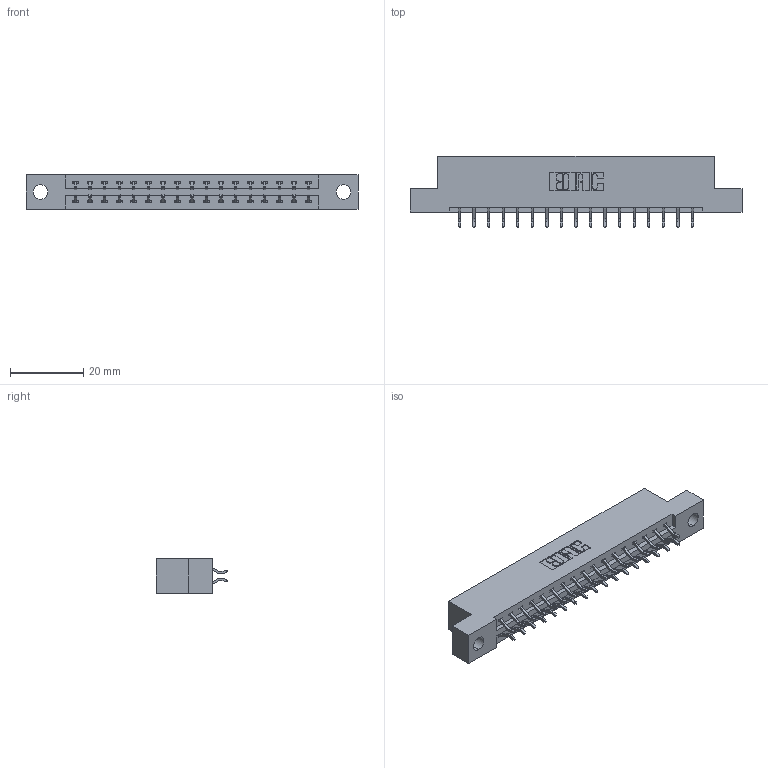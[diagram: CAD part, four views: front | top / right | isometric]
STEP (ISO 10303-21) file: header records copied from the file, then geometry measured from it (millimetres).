
FILE_DESCRIPTION (( 'STEP AP203' ), '1' );
FILE_NAME ('387-034-556-204.STEP', '2018-09-18T21:13:54', ( '' ), ( '' ), 'SwSTEP 2.0', 'SolidWorks 2016', '' );
FILE_SCHEMA (( 'CONFIG_CONTROL_DESIGN' ));
Length unit declared in the file: inch
Products named in the file (3): 387-034-556-204; 337 Part_Flush Mounting Lugs - 0.156 Dia-TH; 345-292-001_556 Tail
Assembly tree (35 placements, depth 2):
  387-034-556-204
    337 Part_Flush Mounting Lugs - 0.156 Dia-TH
    345-292-001_556 Tail  x34
Bounding box: 90.37 x 19.57 x 9.4 mm (x, y, z)
Volume: 9102.3 mm3; surface area: 9808.8 mm2
Topology: 35 solids, 35 shells, 2154 faces, 6397 edges, 4218 vertices
Faces by surface type: plane 1498, cylinder 656
Entity records: 16637 total; most frequent: CARTESIAN_POINT 2838, ORIENTED_EDGE 2762, DIRECTION 2449, EDGE_CURVE 1381, LINE 1245, VECTOR 1245, VERTEX_POINT 918, AXIS2_PLACEMENT_3D 602
